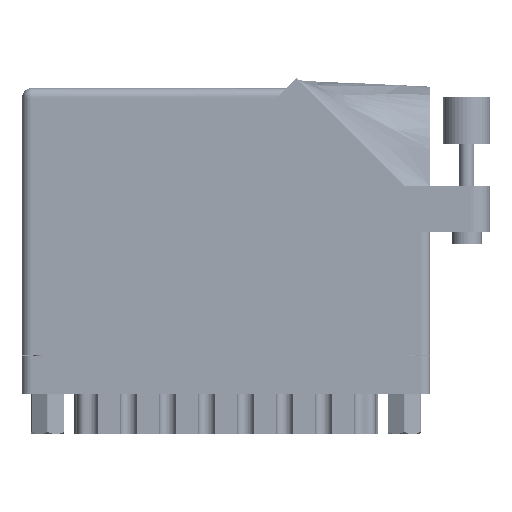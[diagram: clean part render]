
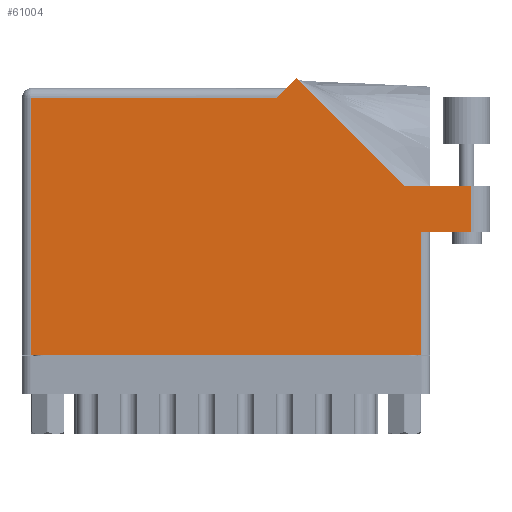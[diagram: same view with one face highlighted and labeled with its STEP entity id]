
A CAD part, front view. The second image highlights one B-rep face of the part: STEP entity #61004.
In plain terms, the highlighted face is planar.
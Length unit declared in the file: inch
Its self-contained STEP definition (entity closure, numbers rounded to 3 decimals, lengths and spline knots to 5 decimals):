
#1149 = VECTOR ( 'NONE', #85657, 39.37008 ) ;
#1458 = VERTEX_POINT ( 'NONE', #51682 ) ;
#2077 = CARTESIAN_POINT ( 'NONE',  ( 1.82871, 1.84571, 0. ) ) ;
#3176 = EDGE_CURVE ( 'NONE', #5472, #5785, #42346, .T. ) ;
#5472 = VERTEX_POINT ( 'NONE', #54059 ) ;
#5785 = VERTEX_POINT ( 'NONE', #49696 ) ;
#6787 = CARTESIAN_POINT ( 'NONE',  ( 2.55242, 1.122, 0. ) ) ;
#7029 = LINE ( 'NONE', #40548, #11320 ) ;
#7643 = CARTESIAN_POINT ( 'NONE',  ( 3.118, 1.122, 0. ) ) ;
#8867 = CARTESIAN_POINT ( 'NONE',  ( 0.062, 0., 0. ) ) ;
#9547 = CARTESIAN_POINT ( 'NONE',  ( 2.993, 0.815, 0. ) ) ;
#10100 = VECTOR ( 'NONE', #74748, 39.37008 ) ;
#11320 = VECTOR ( 'NONE', #72787, 39.37008 ) ;
#11395 = ORIENTED_EDGE ( 'NONE', *, *, #39652, .T. ) ;
#12102 = ORIENTED_EDGE ( 'NONE', *, *, #58207, .T. ) ;
#12483 = EDGE_CURVE ( 'NONE', #1458, #61185, #13652, .T. ) ;
#13652 = LINE ( 'NONE', #58726, #1149 ) ;
#15643 = EDGE_CURVE ( 'NONE', #69239, #78297, #37187, .T. ) ;
#15823 = AXIS2_PLACEMENT_3D ( 'NONE', #37027, #62585, #16627 ) ;
#16041 = PLANE ( 'NONE',  #15823 ) ;
#16627 = DIRECTION ( 'NONE',  ( -1., 0., 0. ) ) ;
#16670 = ORIENTED_EDGE ( 'NONE', *, *, #36049, .T. ) ;
#16895 = LINE ( 'NONE', #53683, #25294 ) ;
#17183 = VERTEX_POINT ( 'NONE', #62842 ) ;
#18363 = LINE ( 'NONE', #53359, #72487 ) ;
#18584 = ORIENTED_EDGE ( 'NONE', *, *, #15643, .T. ) ;
#20399 = CARTESIAN_POINT ( 'NONE',  ( 1.758, 1.775, 0. ) ) ;
#25294 = VECTOR ( 'NONE', #67620, 39.37008 ) ;
#25643 = VERTEX_POINT ( 'NONE', #42176 ) ;
#29770 = EDGE_CURVE ( 'NONE', #78297, #25643, #62579, .T. ) ;
#30582 = VECTOR ( 'NONE', #80299, 39.37008 ) ;
#31748 = CARTESIAN_POINT ( 'NONE',  ( 2.656, 0., 0. ) ) ;
#33502 = DIRECTION ( 'NONE',  ( -1., 0., 0. ) ) ;
#33881 = EDGE_CURVE ( 'NONE', #61185, #17183, #18363, .T. ) ;
#34367 = DIRECTION ( 'NONE',  ( -0.707, -0.707, 0. ) ) ;
#35446 = ORIENTED_EDGE ( 'NONE', *, *, #29770, .T. ) ;
#36049 = EDGE_CURVE ( 'NONE', #5785, #69239, #83568, .T. ) ;
#37027 = CARTESIAN_POINT ( 'NONE',  ( 0., 1.775, 0. ) ) ;
#37187 = LINE ( 'NONE', #20399, #61061 ) ;
#38891 = EDGE_LOOP ( 'NONE', ( #12102, #11395, #50067, #16670, #18584, #35446, #58355, #39072, #69178 ) ) ;
#39072 = ORIENTED_EDGE ( 'NONE', *, *, #12483, .T. ) ;
#39652 = EDGE_CURVE ( 'NONE', #41794, #5472, #7029, .T. ) ;
#40548 = CARTESIAN_POINT ( 'NONE',  ( 2.993, 1.122, 0. ) ) ;
#41794 = VERTEX_POINT ( 'NONE', #9547 ) ;
#42176 = CARTESIAN_POINT ( 'NONE',  ( 0.062, 1.713, 0. ) ) ;
#42346 = LINE ( 'NONE', #7643, #10100 ) ;
#44910 = VECTOR ( 'NONE', #33502, 39.37008 ) ;
#49696 = CARTESIAN_POINT ( 'NONE',  ( 2.55242, 1.122, 0. ) ) ;
#50067 = ORIENTED_EDGE ( 'NONE', *, *, #3176, .T. ) ;
#51682 = CARTESIAN_POINT ( 'NONE',  ( 0.062, 0., 0. ) ) ;
#53359 = CARTESIAN_POINT ( 'NONE',  ( 2.656, 0.815, 0. ) ) ;
#53461 = EDGE_CURVE ( 'NONE', #25643, #1458, #54447, .T. ) ;
#53683 = CARTESIAN_POINT ( 'NONE',  ( 2.718, 0.815, 0. ) ) ;
#54059 = CARTESIAN_POINT ( 'NONE',  ( 2.993, 1.122, 0. ) ) ;
#54447 = LINE ( 'NONE', #8867, #58652 ) ;
#58207 = EDGE_CURVE ( 'NONE', #17183, #41794, #16895, .T. ) ;
#58355 = ORIENTED_EDGE ( 'NONE', *, *, #53461, .T. ) ;
#58652 = VECTOR ( 'NONE', #75424, 39.37008 ) ;
#58726 = CARTESIAN_POINT ( 'NONE',  ( 0., 0., 0. ) ) ;
#61004 = ADVANCED_FACE ( 'NONE', ( #78811 ), #16041, .F. ) ;
#61061 = VECTOR ( 'NONE', #34367, 39.37008 ) ;
#61185 = VERTEX_POINT ( 'NONE', #31748 ) ;
#62579 = LINE ( 'NONE', #79714, #44910 ) ;
#62585 = DIRECTION ( 'NONE',  ( 0., 0., -1. ) ) ;
#62842 = CARTESIAN_POINT ( 'NONE',  ( 2.656, 0.815, 0. ) ) ;
#66985 = DIRECTION ( 'NONE',  ( 0., 1., 0. ) ) ;
#67620 = DIRECTION ( 'NONE',  ( 1., 0., 0. ) ) ;
#69178 = ORIENTED_EDGE ( 'NONE', *, *, #33881, .T. ) ;
#69239 = VERTEX_POINT ( 'NONE', #2077 ) ;
#71426 = CARTESIAN_POINT ( 'NONE',  ( 1.696, 1.713, 0. ) ) ;
#72487 = VECTOR ( 'NONE', #66985, 39.37008 ) ;
#72787 = DIRECTION ( 'NONE',  ( 0., 1., 0. ) ) ;
#74748 = DIRECTION ( 'NONE',  ( -1., 0., 0. ) ) ;
#75424 = DIRECTION ( 'NONE',  ( 0., -1., 0. ) ) ;
#78297 = VERTEX_POINT ( 'NONE', #71426 ) ;
#78811 = FACE_OUTER_BOUND ( 'NONE', #38891, .T. ) ;
#79714 = CARTESIAN_POINT ( 'NONE',  ( 0., 1.713, 0. ) ) ;
#80299 = DIRECTION ( 'NONE',  ( -0.707, 0.707, 0. ) ) ;
#83568 = LINE ( 'NONE', #6787, #30582 ) ;
#85657 = DIRECTION ( 'NONE',  ( 1., 0., 0. ) ) ;
